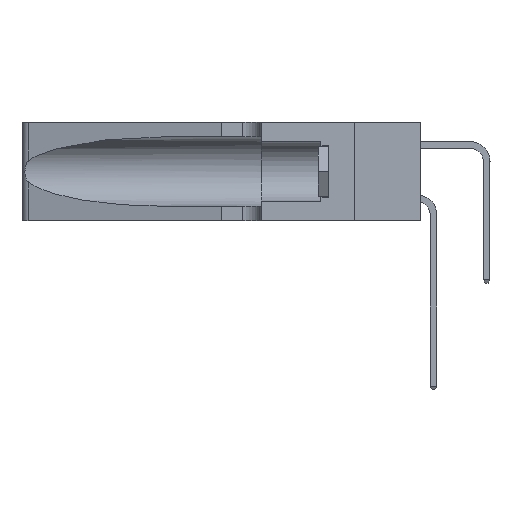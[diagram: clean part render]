
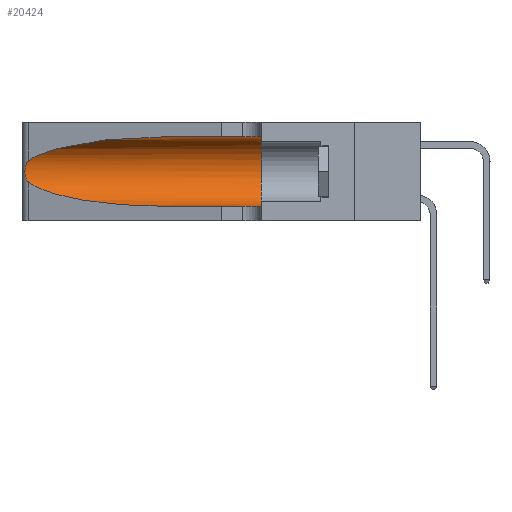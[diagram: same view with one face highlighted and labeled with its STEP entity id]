
A CAD part, left-side view. The second image highlights one B-rep face of the part: STEP entity #20424.
In plain terms, the highlighted cylindrical face has radius 3.308 mm (diameter 6.617 mm), a partial arc.
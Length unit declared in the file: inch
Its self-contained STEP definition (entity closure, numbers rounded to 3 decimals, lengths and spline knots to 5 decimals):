
#133 = CIRCLE ( 'NONE', #22323, 0.13025 ) ;
#235 = CARTESIAN_POINT ( 'NONE',  ( 0.1305, 0.72297, 0.05475 ) ) ;
#1122 = DIRECTION ( 'NONE',  ( 0., 0., -1. ) ) ;
#1405 = CARTESIAN_POINT ( 'NONE',  ( 0.25555, 1.22994, 0.2215 ) ) ;
#2179 = ORIENTED_EDGE ( 'NONE', *, *, #16871, .T. ) ;
#2213 = VERTEX_POINT ( 'NONE', #235 ) ;
#2392 = CARTESIAN_POINT ( 'NONE',  ( 0.2373, 1.15595, 0.28018 ) ) ;
#2798 = CARTESIAN_POINT ( 'NONE',  ( 0.25487, 1.22718, 0.14631 ) ) ;
#2868 = DIRECTION ( 'NONE',  ( 0., -1., 0. ) ) ;
#3319 = CARTESIAN_POINT ( 'NONE',  ( 0.25789, 1.23486, 0.15765 ) ) ;
#3406 = CARTESIAN_POINT ( 'NONE',  ( 0.26075, 1.23896, 0.19203 ) ) ;
#3570 = CARTESIAN_POINT ( 'NONE',  ( 0.25639, 1.23184, 0.21858 ) ) ;
#4268 = EDGE_CURVE ( 'NONE', #20356, #23402, #5856, .T. ) ;
#5212 = CARTESIAN_POINT ( 'NONE',  ( 0.25487, 1.22718, 0.14631 ) ) ;
#5322 = VERTEX_POINT ( 'NONE', #24565 ) ;
#5597 = ORIENTED_EDGE ( 'NONE', *, *, #4268, .T. ) ;
#5856 = B_SPLINE_CURVE_WITH_KNOTS ( 'NONE', 3,
 ( #23094, #1405, #3570, #25127, #15245, #15157, #3406, #13513, #17329, #23269, #3319, #17415, #21346, #5212 ),
 .UNSPECIFIED., .F., .F.,
 ( 4, 2, 2, 2, 2, 2, 4 ),
 ( 0., 0.00027, 0.00053, 0.00107, 0.0016, 0.00187, 0.00214 ),
 .UNSPECIFIED. ) ;
#6927 = CARTESIAN_POINT ( 'NONE',  ( 0.1305, 0.72297, 0.31525 ) ) ;
#6968 =( BOUNDED_CURVE ( )  B_SPLINE_CURVE ( 3, ( #21995, #14225, #2392, #23852 ),
 .UNSPECIFIED., .F., .T. ) 
 B_SPLINE_CURVE_WITH_KNOTS ( ( 4, 4 ),
 ( 1.5708, 2.84003 ),
 .UNSPECIFIED. ) 
 CURVE ( )  GEOMETRIC_REPRESENTATION_ITEM ( )  RATIONAL_B_SPLINE_CURVE ( ( 1., 0.87, 0.87, 1. ) ) 
 REPRESENTATION_ITEM ( '' )  );
#8247 = AXIS2_PLACEMENT_3D ( 'NONE', #14334, #20452, #1122 ) ;
#8635 = CARTESIAN_POINT ( 'NONE',  ( 0.2373, 1.15595, 0.08982 ) ) ;
#8643 = CYLINDRICAL_SURFACE ( 'NONE', #8247, 0.13025 ) ;
#8961 = EDGE_CURVE ( 'NONE', #2213, #18018, #23933, .T. ) ;
#9179 = VERTEX_POINT ( 'NONE', #6927 ) ;
#10799 = EDGE_CURVE ( 'NONE', #23402, #2213, #18063, .T. ) ;
#12991 = ORIENTED_EDGE ( 'NONE', *, *, #13444, .F. ) ;
#13444 = EDGE_CURVE ( 'NONE', #9179, #5322, #23671, .T. ) ;
#13513 = CARTESIAN_POINT ( 'NONE',  ( 0.26075, 1.23896, 0.178 ) ) ;
#13923 = CARTESIAN_POINT ( 'NONE',  ( 0.25487, 1.22718, 0.22369 ) ) ;
#14225 = CARTESIAN_POINT ( 'NONE',  ( 0.18966, 0.96281, 0.31525 ) ) ;
#14334 = CARTESIAN_POINT ( 'NONE',  ( 0.1305, 1.61858, 0.185 ) ) ;
#14488 = CARTESIAN_POINT ( 'NONE',  ( 0.1305, 0.72297, 0.05475 ) ) ;
#15157 = CARTESIAN_POINT ( 'NONE',  ( 0.26018, 1.23835, 0.19895 ) ) ;
#15245 = CARTESIAN_POINT ( 'NONE',  ( 0.25854, 1.2359, 0.20912 ) ) ;
#16442 = ORIENTED_EDGE ( 'NONE', *, *, #8961, .T. ) ;
#16528 = EDGE_CURVE ( 'NONE', #5322, #18018, #133, .T. ) ;
#16871 = EDGE_CURVE ( 'NONE', #9179, #20356, #6968, .T. ) ;
#17329 = CARTESIAN_POINT ( 'NONE',  ( 0.26017, 1.23833, 0.17102 ) ) ;
#17415 = CARTESIAN_POINT ( 'NONE',  ( 0.25639, 1.23186, 0.15144 ) ) ;
#17668 = VECTOR ( 'NONE', #2868, 39.37008 ) ;
#18018 = VERTEX_POINT ( 'NONE', #24167 ) ;
#18063 =( BOUNDED_CURVE ( )  B_SPLINE_CURVE ( 3, ( #20512, #8635, #18648, #14488 ),
 .UNSPECIFIED., .F., .F. ) 
 B_SPLINE_CURVE_WITH_KNOTS ( ( 4, 4 ),
 ( 3.44316, 4.71239 ),
 .UNSPECIFIED. ) 
 CURVE ( )  GEOMETRIC_REPRESENTATION_ITEM ( )  RATIONAL_B_SPLINE_CURVE ( ( 1., 0.87, 0.87, 1. ) ) 
 REPRESENTATION_ITEM ( '' )  );
#18648 = CARTESIAN_POINT ( 'NONE',  ( 0.18966, 0.96281, 0.05475 ) ) ;
#20356 = VERTEX_POINT ( 'NONE', #13923 ) ;
#20424 = ADVANCED_FACE ( 'NONE', ( #22180 ), #8643, .F. ) ;
#20452 = DIRECTION ( 'NONE',  ( 0., -1., 0. ) ) ;
#20512 = CARTESIAN_POINT ( 'NONE',  ( 0.25487, 1.22718, 0.14631 ) ) ;
#20579 = EDGE_LOOP ( 'NONE', ( #2179, #5597, #20929, #16442, #25695, #12991 ) ) ;
#20929 = ORIENTED_EDGE ( 'NONE', *, *, #10799, .T. ) ;
#21346 = CARTESIAN_POINT ( 'NONE',  ( 0.25555, 1.22993, 0.14849 ) ) ;
#21783 = VECTOR ( 'NONE', #24269, 39.37008 ) ;
#21995 = CARTESIAN_POINT ( 'NONE',  ( 0.1305, 0.72297, 0.31525 ) ) ;
#22180 = FACE_OUTER_BOUND ( 'NONE', #20579, .T. ) ;
#22323 = AXIS2_PLACEMENT_3D ( 'NONE', #22418, #24372, #24463 ) ;
#22418 = CARTESIAN_POINT ( 'NONE',  ( 0.1305, 0.35, 0.185 ) ) ;
#22561 = CARTESIAN_POINT ( 'NONE',  ( 0.1305, 1.61858, 0.05475 ) ) ;
#23094 = CARTESIAN_POINT ( 'NONE',  ( 0.25487, 1.22718, 0.22369 ) ) ;
#23269 = CARTESIAN_POINT ( 'NONE',  ( 0.25856, 1.23593, 0.16098 ) ) ;
#23402 = VERTEX_POINT ( 'NONE', #2798 ) ;
#23671 = LINE ( 'NONE', #25395, #21783 ) ;
#23852 = CARTESIAN_POINT ( 'NONE',  ( 0.25487, 1.22718, 0.22369 ) ) ;
#23933 = LINE ( 'NONE', #22561, #17668 ) ;
#24167 = CARTESIAN_POINT ( 'NONE',  ( 0.1305, 0.35, 0.05475 ) ) ;
#24269 = DIRECTION ( 'NONE',  ( 0., -1., 0. ) ) ;
#24372 = DIRECTION ( 'NONE',  ( 0., 1., 0. ) ) ;
#24463 = DIRECTION ( 'NONE',  ( 0., 0., 1. ) ) ;
#24565 = CARTESIAN_POINT ( 'NONE',  ( 0.1305, 0.35, 0.31525 ) ) ;
#25127 = CARTESIAN_POINT ( 'NONE',  ( 0.25787, 1.23484, 0.2124 ) ) ;
#25395 = CARTESIAN_POINT ( 'NONE',  ( 0.1305, 1.61858, 0.31525 ) ) ;
#25695 = ORIENTED_EDGE ( 'NONE', *, *, #16528, .F. ) ;
